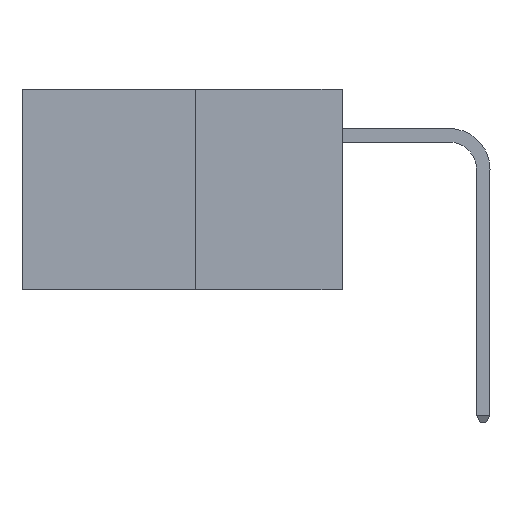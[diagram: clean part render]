
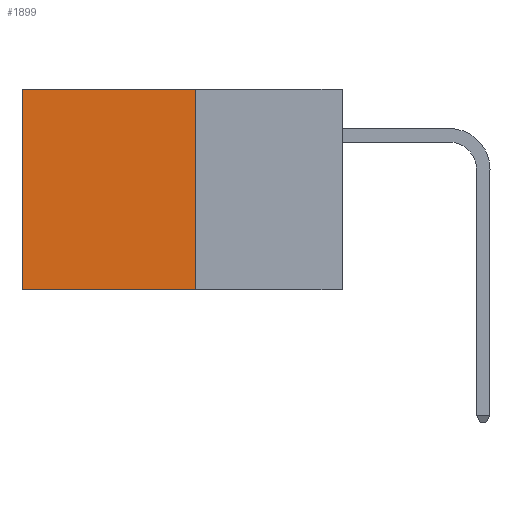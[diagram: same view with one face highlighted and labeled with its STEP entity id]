
A CAD part, left-side view. The second image highlights one B-rep face of the part: STEP entity #1899.
In plain terms, the highlighted planar face has unit normal (-1, 0, 0).
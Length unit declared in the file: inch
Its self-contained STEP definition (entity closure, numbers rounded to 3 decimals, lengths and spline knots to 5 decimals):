
#1899 = ADVANCED_FACE ( 'NONE', ( #6211 ), #13937, .F. ) ;
#2088 = VECTOR ( 'NONE', #9110, 39.37008 ) ;
#3261 = VERTEX_POINT ( 'NONE', #3443 ) ;
#3406 = VERTEX_POINT ( 'NONE', #11277 ) ;
#3443 = CARTESIAN_POINT ( 'NONE',  ( 0.277, 0.27, -0.37 ) ) ;
#4453 = ORIENTED_EDGE ( 'NONE', *, *, #17267, .T. ) ;
#4816 = CARTESIAN_POINT ( 'NONE',  ( 0.277, 0.27, -0.37 ) ) ;
#4891 = ORIENTED_EDGE ( 'NONE', *, *, #16020, .F. ) ;
#4906 = VECTOR ( 'NONE', #16391, 39.37008 ) ;
#6211 = FACE_OUTER_BOUND ( 'NONE', #11306, .T. ) ;
#6445 = CARTESIAN_POINT ( 'NONE',  ( 0.277, 0.59, 0. ) ) ;
#7504 = CARTESIAN_POINT ( 'NONE',  ( 0.277, 0.27, -0.37 ) ) ;
#8301 = DIRECTION ( 'NONE',  ( 1., 0., 0. ) ) ;
#8914 = DIRECTION ( 'NONE',  ( 0., 1., 0. ) ) ;
#9041 = LINE ( 'NONE', #17047, #2088 ) ;
#9110 = DIRECTION ( 'NONE',  ( 0., 0., -1. ) ) ;
#9165 = AXIS2_PLACEMENT_3D ( 'NONE', #4816, #8301, #15252 ) ;
#9801 = EDGE_CURVE ( 'NONE', #3406, #16783, #15717, .T. ) ;
#10181 = EDGE_CURVE ( 'NONE', #3406, #3261, #13008, .T. ) ;
#10708 = DIRECTION ( 'NONE',  ( 0., 0., -1. ) ) ;
#11277 = CARTESIAN_POINT ( 'NONE',  ( 0.277, 0.27, 0. ) ) ;
#11306 = EDGE_LOOP ( 'NONE', ( #4453, #4891, #12594, #16509 ) ) ;
#11645 = LINE ( 'NONE', #7504, #14355 ) ;
#12588 = VECTOR ( 'NONE', #10708, 39.37008 ) ;
#12594 = ORIENTED_EDGE ( 'NONE', *, *, #10181, .F. ) ;
#12666 = VERTEX_POINT ( 'NONE', #14289 ) ;
#13008 = LINE ( 'NONE', #14657, #12588 ) ;
#13937 = PLANE ( 'NONE',  #9165 ) ;
#14289 = CARTESIAN_POINT ( 'NONE',  ( 0.277, 0.59, -0.37 ) ) ;
#14355 = VECTOR ( 'NONE', #8914, 39.37008 ) ;
#14657 = CARTESIAN_POINT ( 'NONE',  ( 0.277, 0.27, -0.37 ) ) ;
#15078 = CARTESIAN_POINT ( 'NONE',  ( 0.277, 0.27, 0. ) ) ;
#15252 = DIRECTION ( 'NONE',  ( 0., 0., -1. ) ) ;
#15717 = LINE ( 'NONE', #15078, #4906 ) ;
#16020 = EDGE_CURVE ( 'NONE', #3261, #12666, #11645, .T. ) ;
#16391 = DIRECTION ( 'NONE',  ( 0., 1., 0. ) ) ;
#16509 = ORIENTED_EDGE ( 'NONE', *, *, #9801, .T. ) ;
#16783 = VERTEX_POINT ( 'NONE', #6445 ) ;
#17047 = CARTESIAN_POINT ( 'NONE',  ( 0.277, 0.59, -0.37 ) ) ;
#17267 = EDGE_CURVE ( 'NONE', #16783, #12666, #9041, .T. ) ;
